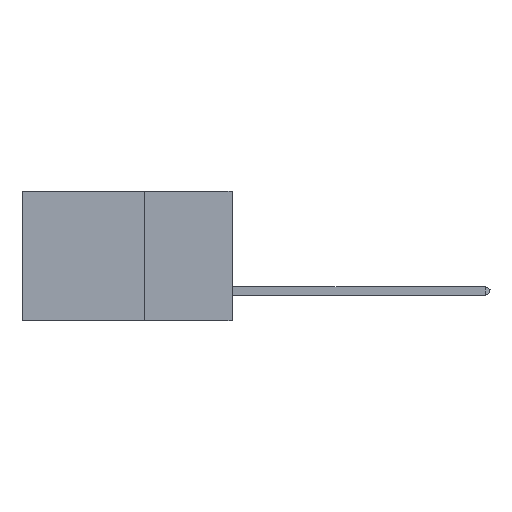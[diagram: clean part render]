
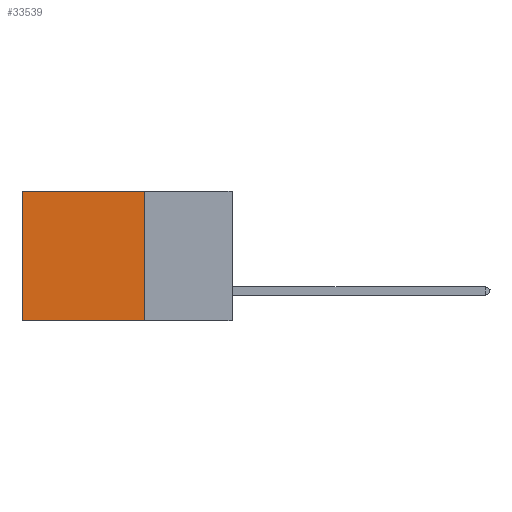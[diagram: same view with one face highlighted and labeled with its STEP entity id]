
A CAD part, left-side view. The second image highlights one B-rep face of the part: STEP entity #33539.
In plain terms, the highlighted planar face has unit normal (-1, 0, 0).
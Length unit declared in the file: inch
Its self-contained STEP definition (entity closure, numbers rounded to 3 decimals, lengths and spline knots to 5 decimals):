
#1137 = CARTESIAN_POINT ( 'NONE',  ( 0.2875, 0.6, 0. ) ) ;
#3811 = ORIENTED_EDGE ( 'NONE', *, *, #29711, .F. ) ;
#4604 = CARTESIAN_POINT ( 'NONE',  ( 0.2875, 0.25, -0.37 ) ) ;
#6095 = DIRECTION ( 'NONE',  ( 0., 0., -1. ) ) ;
#7941 = EDGE_LOOP ( 'NONE', ( #17752, #39880, #3811, #30419 ) ) ;
#9152 = EDGE_CURVE ( 'NONE', #36925, #18801, #35655, .T. ) ;
#11562 = EDGE_CURVE ( 'NONE', #25885, #18801, #23615, .T. ) ;
#11759 = DIRECTION ( 'NONE',  ( 0., 1., 0. ) ) ;
#13077 = DIRECTION ( 'NONE',  ( 0., 0., -1. ) ) ;
#15340 = DIRECTION ( 'NONE',  ( 0., 0., -1. ) ) ;
#17151 = CARTESIAN_POINT ( 'NONE',  ( 0.2875, 0.25, 0. ) ) ;
#17752 = ORIENTED_EDGE ( 'NONE', *, *, #9152, .T. ) ;
#18746 = VECTOR ( 'NONE', #6095, 39.37008 ) ;
#18801 = VERTEX_POINT ( 'NONE', #37386 ) ;
#20085 = LINE ( 'NONE', #39303, #25572 ) ;
#21076 = AXIS2_PLACEMENT_3D ( 'NONE', #28042, #21906, #15340 ) ;
#21906 = DIRECTION ( 'NONE',  ( 1., 0., 0. ) ) ;
#23615 = LINE ( 'NONE', #24040, #24609 ) ;
#24040 = CARTESIAN_POINT ( 'NONE',  ( 0.2875, 0.25, -0.37 ) ) ;
#24609 = VECTOR ( 'NONE', #11759, 39.37008 ) ;
#25572 = VECTOR ( 'NONE', #32986, 39.37008 ) ;
#25885 = VERTEX_POINT ( 'NONE', #4604 ) ;
#28042 = CARTESIAN_POINT ( 'NONE',  ( 0.2875, 0.25, 0. ) ) ;
#28180 = PLANE ( 'NONE',  #21076 ) ;
#29711 = EDGE_CURVE ( 'NONE', #30226, #25885, #31049, .T. ) ;
#30226 = VERTEX_POINT ( 'NONE', #17151 ) ;
#30419 = ORIENTED_EDGE ( 'NONE', *, *, #35567, .T. ) ;
#31049 = LINE ( 'NONE', #31981, #35981 ) ;
#31981 = CARTESIAN_POINT ( 'NONE',  ( 0.2875, 0.25, 0. ) ) ;
#32986 = DIRECTION ( 'NONE',  ( 0., 1., 0. ) ) ;
#33539 = ADVANCED_FACE ( 'NONE', ( #37721 ), #28180, .F. ) ;
#34123 = CARTESIAN_POINT ( 'NONE',  ( 0.2875, 0.6, 0. ) ) ;
#35567 = EDGE_CURVE ( 'NONE', #30226, #36925, #20085, .T. ) ;
#35655 = LINE ( 'NONE', #34123, #18746 ) ;
#35981 = VECTOR ( 'NONE', #13077, 39.37008 ) ;
#36925 = VERTEX_POINT ( 'NONE', #1137 ) ;
#37386 = CARTESIAN_POINT ( 'NONE',  ( 0.2875, 0.6, -0.37 ) ) ;
#37721 = FACE_OUTER_BOUND ( 'NONE', #7941, .T. ) ;
#39303 = CARTESIAN_POINT ( 'NONE',  ( 0.2875, 0.25, 0. ) ) ;
#39880 = ORIENTED_EDGE ( 'NONE', *, *, #11562, .F. ) ;
